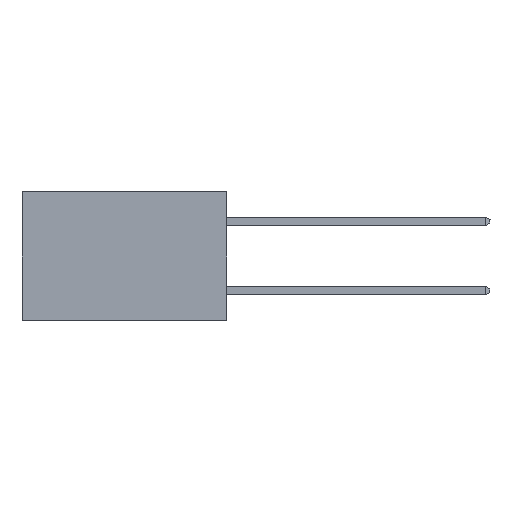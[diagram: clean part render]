
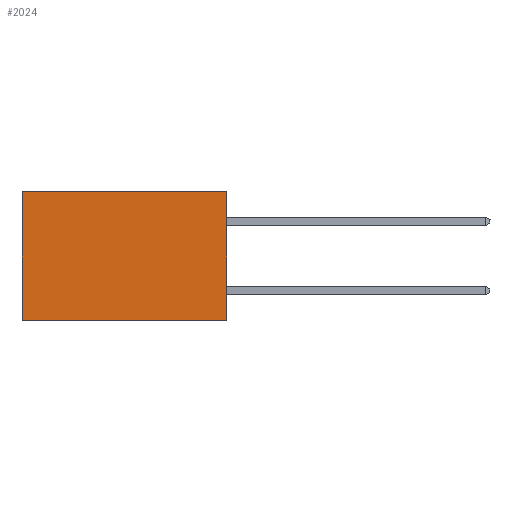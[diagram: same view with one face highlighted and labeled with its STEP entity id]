
A CAD part, left-side view. The second image highlights one B-rep face of the part: STEP entity #2024.
In plain terms, the highlighted planar face has unit normal (-1, 0, 0).
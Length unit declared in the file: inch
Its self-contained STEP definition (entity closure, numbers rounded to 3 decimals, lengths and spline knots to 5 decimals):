
#538 = CARTESIAN_POINT ( 'NONE',  ( 0.277, 0., -0.37 ) ) ;
#1113 = CARTESIAN_POINT ( 'NONE',  ( 0.277, 0., 0. ) ) ;
#1375 = LINE ( 'NONE', #18403, #6099 ) ;
#1893 = VECTOR ( 'NONE', #7307, 39.37008 ) ;
#2024 = ADVANCED_FACE ( 'NONE', ( #13954 ), #17571, .F. ) ;
#2075 = DIRECTION ( 'NONE',  ( 0., 1., 0. ) ) ;
#2386 = DIRECTION ( 'NONE',  ( 0., 0., -1. ) ) ;
#3322 = LINE ( 'NONE', #14563, #24213 ) ;
#4922 = EDGE_CURVE ( 'NONE', #8812, #14791, #17558, .T. ) ;
#6099 = VECTOR ( 'NONE', #2075, 39.37008 ) ;
#6349 = LINE ( 'NONE', #21674, #17295 ) ;
#7206 = CARTESIAN_POINT ( 'NONE',  ( 0.277, 0., -0.37 ) ) ;
#7299 = CARTESIAN_POINT ( 'NONE',  ( 0.277, 0.59, -0.37 ) ) ;
#7307 = DIRECTION ( 'NONE',  ( 0., 0., -1. ) ) ;
#8812 = VERTEX_POINT ( 'NONE', #1113 ) ;
#9197 = EDGE_LOOP ( 'NONE', ( #16057, #16304, #16747, #17297 ) ) ;
#9447 = DIRECTION ( 'NONE',  ( 0., 1., 0. ) ) ;
#11834 = EDGE_CURVE ( 'NONE', #14791, #16509, #1375, .T. ) ;
#13737 = EDGE_CURVE ( 'NONE', #8812, #16835, #6349, .T. ) ;
#13954 = FACE_OUTER_BOUND ( 'NONE', #9197, .T. ) ;
#14563 = CARTESIAN_POINT ( 'NONE',  ( 0.277, 0.59, -0.37 ) ) ;
#14791 = VERTEX_POINT ( 'NONE', #538 ) ;
#16057 = ORIENTED_EDGE ( 'NONE', *, *, #17649, .T. ) ;
#16304 = ORIENTED_EDGE ( 'NONE', *, *, #11834, .F. ) ;
#16509 = VERTEX_POINT ( 'NONE', #7299 ) ;
#16747 = ORIENTED_EDGE ( 'NONE', *, *, #4922, .F. ) ;
#16835 = VERTEX_POINT ( 'NONE', #20357 ) ;
#17295 = VECTOR ( 'NONE', #9447, 39.37008 ) ;
#17297 = ORIENTED_EDGE ( 'NONE', *, *, #13737, .T. ) ;
#17558 = LINE ( 'NONE', #7206, #1893 ) ;
#17571 = PLANE ( 'NONE',  #17878 ) ;
#17649 = EDGE_CURVE ( 'NONE', #16835, #16509, #3322, .T. ) ;
#17878 = AXIS2_PLACEMENT_3D ( 'NONE', #22096, #23744, #18759 ) ;
#18403 = CARTESIAN_POINT ( 'NONE',  ( 0.277, 0., -0.37 ) ) ;
#18759 = DIRECTION ( 'NONE',  ( 0., 0., -1. ) ) ;
#20357 = CARTESIAN_POINT ( 'NONE',  ( 0.277, 0.59, 0. ) ) ;
#21674 = CARTESIAN_POINT ( 'NONE',  ( 0.277, 0., 0. ) ) ;
#22096 = CARTESIAN_POINT ( 'NONE',  ( 0.277, 0., -0.37 ) ) ;
#23744 = DIRECTION ( 'NONE',  ( 1., 0., 0. ) ) ;
#24213 = VECTOR ( 'NONE', #2386, 39.37008 ) ;
